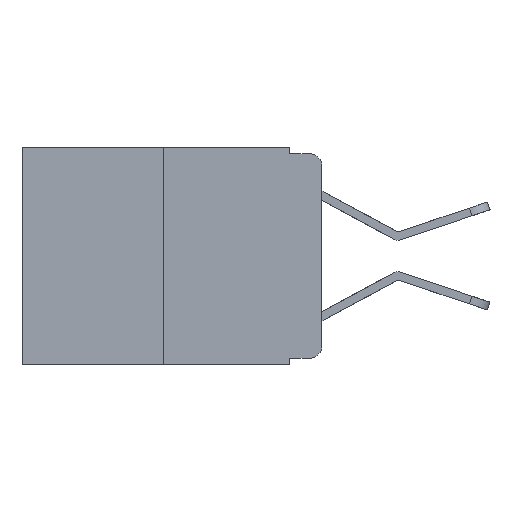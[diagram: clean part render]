
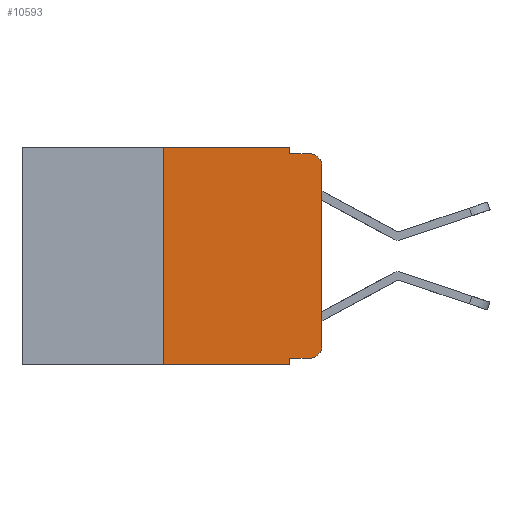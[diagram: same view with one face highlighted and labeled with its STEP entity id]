
A CAD part, left-side view. The second image highlights one B-rep face of the part: STEP entity #10593.
In plain terms, the highlighted planar face has unit normal (-1, 0, 0).
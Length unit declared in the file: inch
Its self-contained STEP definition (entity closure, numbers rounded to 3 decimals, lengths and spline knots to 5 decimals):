
#46 = DIRECTION ( 'NONE',  ( -1., 0., 0. ) ) ;
#315 = ORIENTED_EDGE ( 'NONE', *, *, #10168, .F. ) ;
#388 = EDGE_LOOP ( 'NONE', ( #1718, #6043, #9980, #11972, #315, #7771, #6565, #16802, #12746, #13217 ) ) ;
#1496 = EDGE_CURVE ( 'NONE', #18263, #2672, #4964, .T. ) ;
#1718 = ORIENTED_EDGE ( 'NONE', *, *, #18440, .T. ) ;
#1912 = VERTEX_POINT ( 'NONE', #19935 ) ;
#2133 = DIRECTION ( 'NONE',  ( 0., -1., 0. ) ) ;
#2306 = EDGE_CURVE ( 'NONE', #20570, #17299, #15785, .T. ) ;
#2383 = CARTESIAN_POINT ( 'NONE',  ( 0., 0.051, -0.333 ) ) ;
#2388 = LINE ( 'NONE', #5009, #6655 ) ;
#2597 = CARTESIAN_POINT ( 'NONE',  ( 0., 0., -0.03 ) ) ;
#2672 = VERTEX_POINT ( 'NONE', #13920 ) ;
#3005 = CARTESIAN_POINT ( 'NONE',  ( 0., 0.02, -0.333 ) ) ;
#3164 = VECTOR ( 'NONE', #20553, 39.37008 ) ;
#3458 = VERTEX_POINT ( 'NONE', #20455 ) ;
#4253 = CARTESIAN_POINT ( 'NONE',  ( 0., 0.051, -0.01 ) ) ;
#4320 = CARTESIAN_POINT ( 'NONE',  ( 0., 0.25, 0. ) ) ;
#4885 = EDGE_CURVE ( 'NONE', #17299, #12697, #15801, .T. ) ;
#4964 = LINE ( 'NONE', #12566, #17031 ) ;
#5009 = CARTESIAN_POINT ( 'NONE',  ( 0., 0.051, 0. ) ) ;
#5573 = EDGE_CURVE ( 'NONE', #20570, #2672, #2388, .T. ) ;
#5815 = DIRECTION ( 'NONE',  ( 0., -1., 0. ) ) ;
#5831 = VERTEX_POINT ( 'NONE', #13544 ) ;
#5866 = CARTESIAN_POINT ( 'NONE',  ( 0., 0.051, -0.333 ) ) ;
#6005 = FACE_OUTER_BOUND ( 'NONE', #388, .T. ) ;
#6043 = ORIENTED_EDGE ( 'NONE', *, *, #11169, .T. ) ;
#6063 = CARTESIAN_POINT ( 'NONE',  ( 0., 0.473, 0. ) ) ;
#6332 = DIRECTION ( 'NONE',  ( 0., 0., 1. ) ) ;
#6565 = ORIENTED_EDGE ( 'NONE', *, *, #1496, .T. ) ;
#6655 = VECTOR ( 'NONE', #14495, 39.37008 ) ;
#6996 = VECTOR ( 'NONE', #18783, 39.37008 ) ;
#7012 = LINE ( 'NONE', #9785, #10264 ) ;
#7099 = CARTESIAN_POINT ( 'NONE',  ( 0., 0.25, -0.343 ) ) ;
#7220 = CIRCLE ( 'NONE', #19659, 0.02 ) ;
#7675 = DIRECTION ( 'NONE',  ( 0., 0., -1. ) ) ;
#7771 = ORIENTED_EDGE ( 'NONE', *, *, #8786, .F. ) ;
#7871 = CARTESIAN_POINT ( 'NONE',  ( 0., 0.051, 0. ) ) ;
#8128 = CARTESIAN_POINT ( 'NONE',  ( 0., 0.02, -0.313 ) ) ;
#8786 = EDGE_CURVE ( 'NONE', #18263, #5831, #9070, .T. ) ;
#9070 = LINE ( 'NONE', #4320, #16872 ) ;
#9444 = EDGE_CURVE ( 'NONE', #3458, #15194, #11246, .T. ) ;
#9643 = AXIS2_PLACEMENT_3D ( 'NONE', #6063, #17053, #7675 ) ;
#9785 = CARTESIAN_POINT ( 'NONE',  ( 0., 0.473, 0. ) ) ;
#9855 = CARTESIAN_POINT ( 'NONE',  ( 0., 0.02, -0.03 ) ) ;
#9980 = ORIENTED_EDGE ( 'NONE', *, *, #19867, .F. ) ;
#10168 = EDGE_CURVE ( 'NONE', #5831, #3458, #7012, .T. ) ;
#10264 = VECTOR ( 'NONE', #20629, 39.37008 ) ;
#10593 = ADVANCED_FACE ( 'NONE', ( #6005 ), #15507, .F. ) ;
#10626 = LINE ( 'NONE', #14854, #17883 ) ;
#10714 = CARTESIAN_POINT ( 'NONE',  ( 0., 0., -0.313 ) ) ;
#10984 = DIRECTION ( 'NONE',  ( -1., 0., 0. ) ) ;
#11169 = EDGE_CURVE ( 'NONE', #19410, #1912, #7220, .T. ) ;
#11246 = LINE ( 'NONE', #7871, #6996 ) ;
#11442 = DIRECTION ( 'NONE',  ( 0., 0., -1. ) ) ;
#11972 = ORIENTED_EDGE ( 'NONE', *, *, #9444, .F. ) ;
#12566 = CARTESIAN_POINT ( 'NONE',  ( 0., 0.473, -0.343 ) ) ;
#12697 = VERTEX_POINT ( 'NONE', #10714 ) ;
#12746 = ORIENTED_EDGE ( 'NONE', *, *, #2306, .T. ) ;
#12981 = AXIS2_PLACEMENT_3D ( 'NONE', #8128, #10984, #16169 ) ;
#13217 = ORIENTED_EDGE ( 'NONE', *, *, #4885, .T. ) ;
#13544 = CARTESIAN_POINT ( 'NONE',  ( 0., 0.25, 0. ) ) ;
#13832 = DIRECTION ( 'NONE',  ( 0., 0., 1. ) ) ;
#13920 = CARTESIAN_POINT ( 'NONE',  ( 0., 0.051, -0.343 ) ) ;
#14495 = DIRECTION ( 'NONE',  ( 0., 0., -1. ) ) ;
#14854 = CARTESIAN_POINT ( 'NONE',  ( 0., 0.051, -0.01 ) ) ;
#15194 = VERTEX_POINT ( 'NONE', #4253 ) ;
#15507 = PLANE ( 'NONE',  #9643 ) ;
#15785 = LINE ( 'NONE', #2383, #3164 ) ;
#15801 = CIRCLE ( 'NONE', #12981, 0.02 ) ;
#16009 = VECTOR ( 'NONE', #6332, 39.37008 ) ;
#16169 = DIRECTION ( 'NONE',  ( 0., 0., -1. ) ) ;
#16802 = ORIENTED_EDGE ( 'NONE', *, *, #5573, .F. ) ;
#16872 = VECTOR ( 'NONE', #13832, 39.37008 ) ;
#17031 = VECTOR ( 'NONE', #5815, 39.37008 ) ;
#17053 = DIRECTION ( 'NONE',  ( 1., 0., 0. ) ) ;
#17299 = VERTEX_POINT ( 'NONE', #3005 ) ;
#17312 = CARTESIAN_POINT ( 'NONE',  ( 0., 0., 0. ) ) ;
#17883 = VECTOR ( 'NONE', #2133, 39.37008 ) ;
#18263 = VERTEX_POINT ( 'NONE', #7099 ) ;
#18440 = EDGE_CURVE ( 'NONE', #12697, #19410, #20574, .T. ) ;
#18783 = DIRECTION ( 'NONE',  ( 0., 0., -1. ) ) ;
#19410 = VERTEX_POINT ( 'NONE', #2597 ) ;
#19659 = AXIS2_PLACEMENT_3D ( 'NONE', #9855, #46, #11442 ) ;
#19867 = EDGE_CURVE ( 'NONE', #15194, #1912, #10626, .T. ) ;
#19935 = CARTESIAN_POINT ( 'NONE',  ( 0., 0.02, -0.01 ) ) ;
#20455 = CARTESIAN_POINT ( 'NONE',  ( 0., 0.051, 0. ) ) ;
#20553 = DIRECTION ( 'NONE',  ( 0., -1., 0. ) ) ;
#20570 = VERTEX_POINT ( 'NONE', #5866 ) ;
#20574 = LINE ( 'NONE', #17312, #16009 ) ;
#20629 = DIRECTION ( 'NONE',  ( 0., -1., 0. ) ) ;
